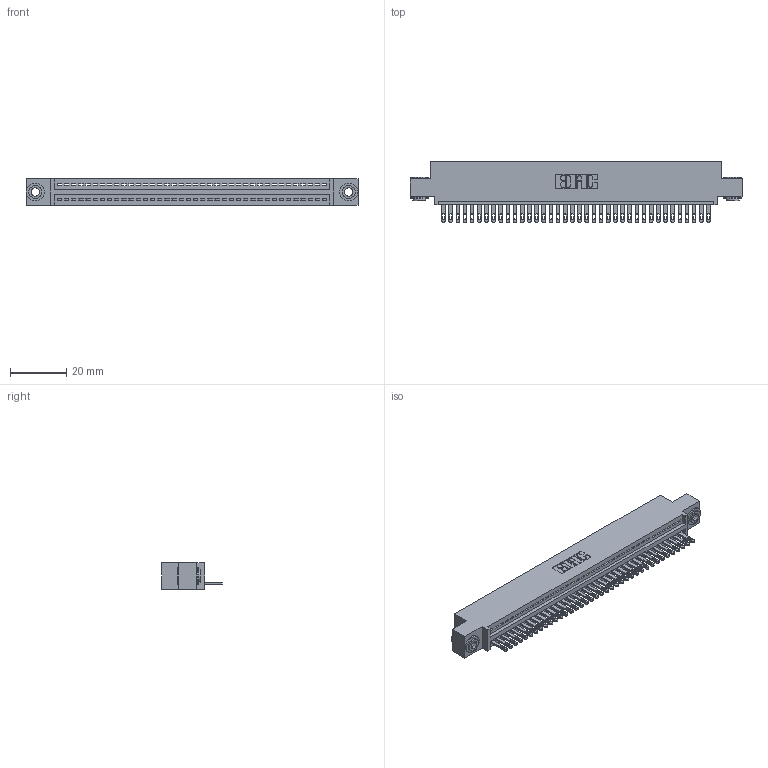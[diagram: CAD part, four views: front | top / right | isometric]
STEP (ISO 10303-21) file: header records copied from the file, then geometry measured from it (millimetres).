
FILE_DESCRIPTION (( 'STEP AP203' ), '1' );
FILE_NAME ('895-038-500-403.STEP', '2020-09-26T00:59:32', ( '' ), ( '' ), 'SwSTEP 2.0', 'SolidWorks 2020', '' );
FILE_SCHEMA (( 'CONFIG_CONTROL_DESIGN' ));
Length unit declared in the file: inch
Products named in the file (4): 345-250-002_345-250-002-102; 895-038-500-403; 845 Part_0.110 Offset - 0.156 Dia-TH; 345-292-001_345-293-100
Assembly tree (41 placements, depth 2):
  895-038-500-403
    845 Part_0.110 Offset - 0.156 Dia-TH
    345-292-001_345-293-100  x38
    345-250-002_345-250-002-102  x2
Bounding box: 117.73 x 21.51 x 9.4 mm (x, y, z)
Volume: 11118.8 mm3; surface area: 15103.2 mm2
Topology: 41 solids, 41 shells, 2220 faces, 6813 edges, 4538 vertices
Faces by surface type: plane 1386, cylinder 826, cone 8
Entity records: 29850 total; most frequent: CARTESIAN_POINT 5149, ORIENTED_EDGE 5114, DIRECTION 4535, EDGE_CURVE 2557, VECTOR 2245, LINE 2245, VERTEX_POINT 1702, AXIS2_PLACEMENT_3D 1145
